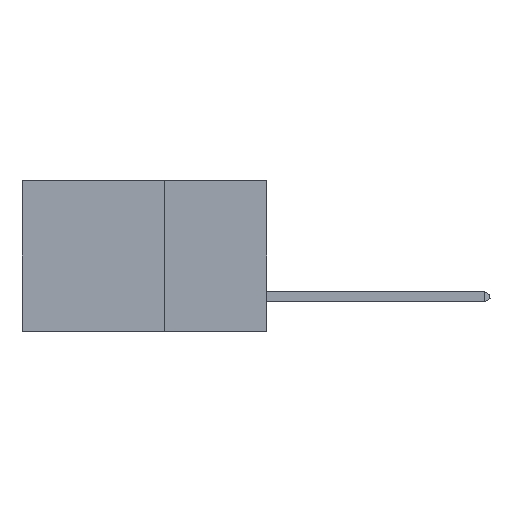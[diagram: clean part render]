
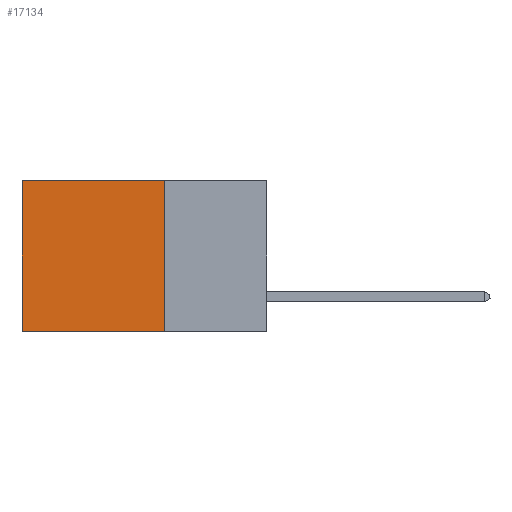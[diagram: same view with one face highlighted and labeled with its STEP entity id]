
A CAD part, left-side view. The second image highlights one B-rep face of the part: STEP entity #17134.
In plain terms, the highlighted planar face has unit normal (-1, 0, 0).
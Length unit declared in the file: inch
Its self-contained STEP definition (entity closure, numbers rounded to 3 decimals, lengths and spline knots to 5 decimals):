
#329 = ORIENTED_EDGE ( 'NONE', *, *, #35856, .F. ) ;
#1005 = EDGE_CURVE ( 'NONE', #18506, #26875, #45660, .T. ) ;
#3792 = DIRECTION ( 'NONE',  ( 0., 0., -1. ) ) ;
#4502 = ORIENTED_EDGE ( 'NONE', *, *, #37482, .T. ) ;
#5000 = VERTEX_POINT ( 'NONE', #36613 ) ;
#7714 = CARTESIAN_POINT ( 'NONE',  ( 0.2875, 0.25, 0. ) ) ;
#10957 = AXIS2_PLACEMENT_3D ( 'NONE', #13538, #43844, #21358 ) ;
#11756 = DIRECTION ( 'NONE',  ( 0., 0., -1. ) ) ;
#13538 = CARTESIAN_POINT ( 'NONE',  ( 0.2875, 0.25, 0. ) ) ;
#14457 = VECTOR ( 'NONE', #44301, 39.37008 ) ;
#14755 = LINE ( 'NONE', #30171, #23642 ) ;
#17134 = ADVANCED_FACE ( 'NONE', ( #20130 ), #17572, .F. ) ;
#17297 = CARTESIAN_POINT ( 'NONE',  ( 0.2875, 0.25, 0. ) ) ;
#17503 = CARTESIAN_POINT ( 'NONE',  ( 0.2875, 0.6, 0. ) ) ;
#17572 = PLANE ( 'NONE',  #10957 ) ;
#17811 = CARTESIAN_POINT ( 'NONE',  ( 0.2875, 0.25, -0.37 ) ) ;
#18041 = CARTESIAN_POINT ( 'NONE',  ( 0.2875, 0.25, 0. ) ) ;
#18506 = VERTEX_POINT ( 'NONE', #17297 ) ;
#20130 = FACE_OUTER_BOUND ( 'NONE', #26518, .T. ) ;
#21358 = DIRECTION ( 'NONE',  ( 0., 0., -1. ) ) ;
#23642 = VECTOR ( 'NONE', #3792, 39.37008 ) ;
#26518 = EDGE_LOOP ( 'NONE', ( #4502, #329, #29280, #39028 ) ) ;
#26875 = VERTEX_POINT ( 'NONE', #36813 ) ;
#28472 = VECTOR ( 'NONE', #44066, 39.37008 ) ;
#29280 = ORIENTED_EDGE ( 'NONE', *, *, #1005, .F. ) ;
#30171 = CARTESIAN_POINT ( 'NONE',  ( 0.2875, 0.6, 0. ) ) ;
#34280 = VERTEX_POINT ( 'NONE', #17503 ) ;
#35856 = EDGE_CURVE ( 'NONE', #26875, #5000, #36087, .T. ) ;
#36087 = LINE ( 'NONE', #17811, #28472 ) ;
#36613 = CARTESIAN_POINT ( 'NONE',  ( 0.2875, 0.6, -0.37 ) ) ;
#36813 = CARTESIAN_POINT ( 'NONE',  ( 0.2875, 0.25, -0.37 ) ) ;
#37482 = EDGE_CURVE ( 'NONE', #34280, #5000, #14755, .T. ) ;
#39028 = ORIENTED_EDGE ( 'NONE', *, *, #48512, .T. ) ;
#43333 = LINE ( 'NONE', #18041, #14457 ) ;
#43844 = DIRECTION ( 'NONE',  ( 1., 0., 0. ) ) ;
#44066 = DIRECTION ( 'NONE',  ( 0., 1., 0. ) ) ;
#44301 = DIRECTION ( 'NONE',  ( 0., 1., 0. ) ) ;
#44506 = VECTOR ( 'NONE', #11756, 39.37008 ) ;
#45660 = LINE ( 'NONE', #7714, #44506 ) ;
#48512 = EDGE_CURVE ( 'NONE', #18506, #34280, #43333, .T. ) ;
